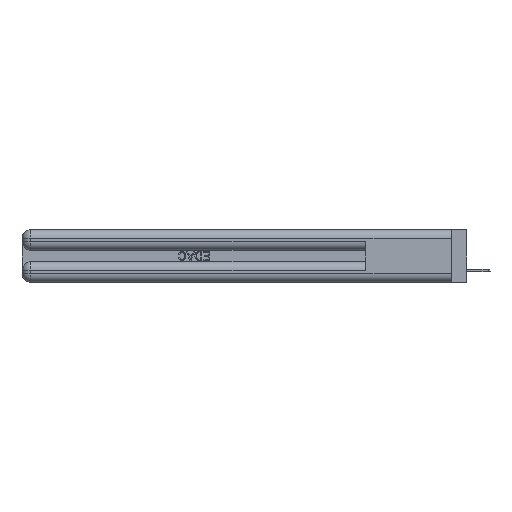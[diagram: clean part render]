
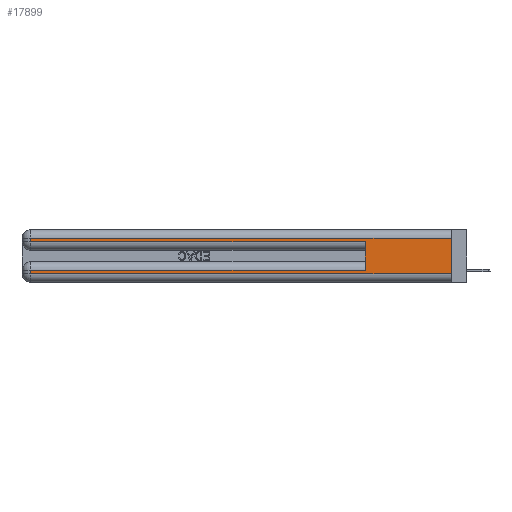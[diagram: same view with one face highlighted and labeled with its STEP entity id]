
A CAD part, left-side view. The second image highlights one B-rep face of the part: STEP entity #17899.
In plain terms, the highlighted planar face has unit normal (-1, 0, 0).
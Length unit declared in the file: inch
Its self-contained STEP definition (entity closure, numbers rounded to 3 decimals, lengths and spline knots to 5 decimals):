
#209 = CARTESIAN_POINT ( 'NONE',  ( 0., 0., 0.31 ) ) ;
#290 = CARTESIAN_POINT ( 'NONE',  ( 0., 0., 0.285 ) ) ;
#761 = CARTESIAN_POINT ( 'NONE',  ( 0., 0.6, 0.085 ) ) ;
#4529 = DIRECTION ( 'NONE',  ( 0., 0., -1. ) ) ;
#6557 = VECTOR ( 'NONE', #42024, 39.37008 ) ;
#6643 = DIRECTION ( 'NONE',  ( 0., 0., 1. ) ) ;
#9620 = DIRECTION ( 'NONE',  ( 0., -1., 0. ) ) ;
#9775 = LINE ( 'NONE', #20530, #19743 ) ;
#9936 = CARTESIAN_POINT ( 'NONE',  ( 0., 2.94, 0.06 ) ) ;
#10476 = DIRECTION ( 'NONE',  ( 0., 1., 0. ) ) ;
#10884 = FACE_OUTER_BOUND ( 'NONE', #28733, .T. ) ;
#12089 = LINE ( 'NONE', #39210, #31360 ) ;
#12613 = CARTESIAN_POINT ( 'NONE',  ( 0., 0.6, 0.285 ) ) ;
#12657 = CARTESIAN_POINT ( 'NONE',  ( 0., 2.94, 0.285 ) ) ;
#12965 = ORIENTED_EDGE ( 'NONE', *, *, #37466, .T. ) ;
#14070 = VERTEX_POINT ( 'NONE', #15846 ) ;
#14447 = DIRECTION ( 'NONE',  ( 1., 0., 0. ) ) ;
#14584 = EDGE_CURVE ( 'NONE', #18517, #14693, #29157, .T. ) ;
#14693 = VERTEX_POINT ( 'NONE', #9936 ) ;
#14988 = AXIS2_PLACEMENT_3D ( 'NONE', #27275, #14447, #24391 ) ;
#15083 = ORIENTED_EDGE ( 'NONE', *, *, #24397, .F. ) ;
#15632 = EDGE_CURVE ( 'NONE', #27320, #18517, #16519, .T. ) ;
#15846 = CARTESIAN_POINT ( 'NONE',  ( 0., 0., 0.06 ) ) ;
#16519 = LINE ( 'NONE', #32130, #6557 ) ;
#17028 = VERTEX_POINT ( 'NONE', #26066 ) ;
#17774 = EDGE_CURVE ( 'NONE', #22558, #17028, #23472, .T. ) ;
#17899 = ADVANCED_FACE ( 'NONE', ( #10884 ), #40627, .F. ) ;
#18517 = VERTEX_POINT ( 'NONE', #38096 ) ;
#19743 = VECTOR ( 'NONE', #42898, 39.37008 ) ;
#19897 = CARTESIAN_POINT ( 'NONE',  ( 0., 2.94, 0.37 ) ) ;
#20019 = EDGE_CURVE ( 'NONE', #27320, #20627, #41436, .T. ) ;
#20113 = ORIENTED_EDGE ( 'NONE', *, *, #20019, .F. ) ;
#20530 = CARTESIAN_POINT ( 'NONE',  ( 0., 0., 0.37 ) ) ;
#20627 = VERTEX_POINT ( 'NONE', #12613 ) ;
#21514 = LINE ( 'NONE', #37608, #36031 ) ;
#22558 = VERTEX_POINT ( 'NONE', #209 ) ;
#23472 = LINE ( 'NONE', #40334, #31257 ) ;
#23829 = DIRECTION ( 'NONE',  ( 0., -1., 0. ) ) ;
#24391 = DIRECTION ( 'NONE',  ( 0., 0., -1. ) ) ;
#24397 = EDGE_CURVE ( 'NONE', #22558, #14070, #9775, .T. ) ;
#26066 = CARTESIAN_POINT ( 'NONE',  ( 0., 2.94, 0.31 ) ) ;
#26568 = VECTOR ( 'NONE', #23829, 39.37008 ) ;
#27275 = CARTESIAN_POINT ( 'NONE',  ( 0., 0., 0.37 ) ) ;
#27320 = VERTEX_POINT ( 'NONE', #761 ) ;
#27532 = EDGE_CURVE ( 'NONE', #14693, #14070, #12089, .T. ) ;
#28158 = ORIENTED_EDGE ( 'NONE', *, *, #15632, .T. ) ;
#28170 = VERTEX_POINT ( 'NONE', #12657 ) ;
#28733 = EDGE_LOOP ( 'NONE', ( #15083, #37839, #38603, #12965, #20113, #28158, #31846, #37898 ) ) ;
#29157 = LINE ( 'NONE', #19897, #34326 ) ;
#31257 = VECTOR ( 'NONE', #10476, 39.37008 ) ;
#31360 = VECTOR ( 'NONE', #9620, 39.37008 ) ;
#31846 = ORIENTED_EDGE ( 'NONE', *, *, #14584, .T. ) ;
#32130 = CARTESIAN_POINT ( 'NONE',  ( 0., 0., 0.085 ) ) ;
#33163 = CARTESIAN_POINT ( 'NONE',  ( 0., 0.6, 0.145 ) ) ;
#34326 = VECTOR ( 'NONE', #39379, 39.37008 ) ;
#35269 = EDGE_CURVE ( 'NONE', #17028, #28170, #21514, .T. ) ;
#36031 = VECTOR ( 'NONE', #4529, 39.37008 ) ;
#36919 = LINE ( 'NONE', #290, #26568 ) ;
#37466 = EDGE_CURVE ( 'NONE', #28170, #20627, #36919, .T. ) ;
#37608 = CARTESIAN_POINT ( 'NONE',  ( 0., 2.94, 0.37 ) ) ;
#37839 = ORIENTED_EDGE ( 'NONE', *, *, #17774, .T. ) ;
#37898 = ORIENTED_EDGE ( 'NONE', *, *, #27532, .T. ) ;
#38096 = CARTESIAN_POINT ( 'NONE',  ( 0., 2.94, 0.085 ) ) ;
#38603 = ORIENTED_EDGE ( 'NONE', *, *, #35269, .T. ) ;
#39210 = CARTESIAN_POINT ( 'NONE',  ( 0., 0., 0.06 ) ) ;
#39379 = DIRECTION ( 'NONE',  ( 0., 0., -1. ) ) ;
#40334 = CARTESIAN_POINT ( 'NONE',  ( 0., 0., 0.31 ) ) ;
#40627 = PLANE ( 'NONE',  #14988 ) ;
#41436 = LINE ( 'NONE', #33163, #41977 ) ;
#41977 = VECTOR ( 'NONE', #6643, 39.37008 ) ;
#42024 = DIRECTION ( 'NONE',  ( 0., 1., 0. ) ) ;
#42898 = DIRECTION ( 'NONE',  ( 0., 0., -1. ) ) ;
